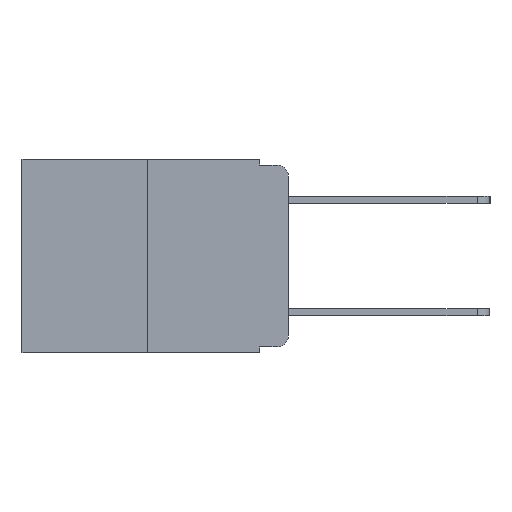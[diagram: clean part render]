
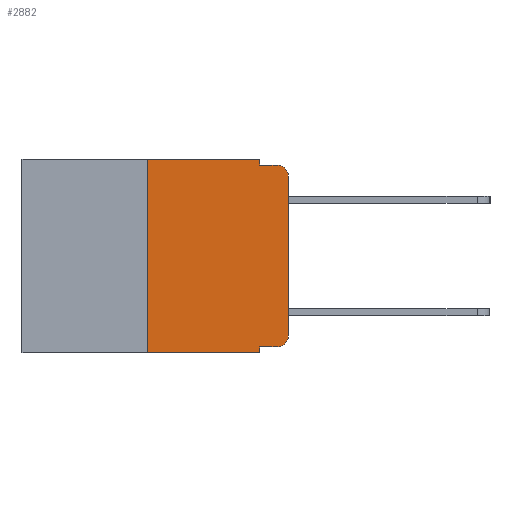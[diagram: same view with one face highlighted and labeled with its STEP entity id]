
A CAD part, left-side view. The second image highlights one B-rep face of the part: STEP entity #2882.
In plain terms, the highlighted planar face has unit normal (-1, 0, 0).
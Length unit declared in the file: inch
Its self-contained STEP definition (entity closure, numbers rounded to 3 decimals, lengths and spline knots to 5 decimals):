
#78 = FACE_OUTER_BOUND ( 'NONE', #7432, .T. ) ;
#578 = CARTESIAN_POINT ( 'NONE',  ( 0., 0.051, -0.343 ) ) ;
#594 = CARTESIAN_POINT ( 'NONE',  ( 0., 0.02, -0.01 ) ) ;
#706 = VECTOR ( 'NONE', #1500, 39.37008 ) ;
#825 = VERTEX_POINT ( 'NONE', #11015 ) ;
#967 = CARTESIAN_POINT ( 'NONE',  ( 0., 0.051, 0. ) ) ;
#990 = LINE ( 'NONE', #9850, #10139 ) ;
#1158 = VECTOR ( 'NONE', #1439, 39.37008 ) ;
#1318 = CARTESIAN_POINT ( 'NONE',  ( 0., 0.051, -0.333 ) ) ;
#1439 = DIRECTION ( 'NONE',  ( 0., -1., 0. ) ) ;
#1500 = DIRECTION ( 'NONE',  ( 0., -1., 0. ) ) ;
#1707 = VERTEX_POINT ( 'NONE', #967 ) ;
#2031 = EDGE_CURVE ( 'NONE', #7863, #6148, #9672, .T. ) ;
#2341 = PLANE ( 'NONE',  #5592 ) ;
#2882 = ADVANCED_FACE ( 'NONE', ( #78 ), #2341, .F. ) ;
#3167 = DIRECTION ( 'NONE',  ( -1., 0., 0. ) ) ;
#3210 = AXIS2_PLACEMENT_3D ( 'NONE', #8360, #3167, #9182 ) ;
#3216 = ORIENTED_EDGE ( 'NONE', *, *, #11448, .F. ) ;
#3262 = EDGE_CURVE ( 'NONE', #6536, #1707, #3329, .T. ) ;
#3329 = LINE ( 'NONE', #3497, #706 ) ;
#3354 = LINE ( 'NONE', #8130, #9667 ) ;
#3497 = CARTESIAN_POINT ( 'NONE',  ( 0., 0.473, 0. ) ) ;
#3505 = ORIENTED_EDGE ( 'NONE', *, *, #2031, .T. ) ;
#3533 = VECTOR ( 'NONE', #6987, 39.37008 ) ;
#3635 = VERTEX_POINT ( 'NONE', #5100 ) ;
#3747 = ORIENTED_EDGE ( 'NONE', *, *, #10014, .T. ) ;
#3861 = DIRECTION ( 'NONE',  ( 0., 0., -1. ) ) ;
#3976 = VECTOR ( 'NONE', #10927, 39.37008 ) ;
#4178 = LINE ( 'NONE', #5050, #8469 ) ;
#4180 = CARTESIAN_POINT ( 'NONE',  ( 0., 0.25, 0. ) ) ;
#4302 = ORIENTED_EDGE ( 'NONE', *, *, #10775, .F. ) ;
#4374 = DIRECTION ( 'NONE',  ( 1., 0., 0. ) ) ;
#4479 = DIRECTION ( 'NONE',  ( -1., 0., 0. ) ) ;
#4480 = CARTESIAN_POINT ( 'NONE',  ( 0., 0.02, -0.313 ) ) ;
#4847 = VERTEX_POINT ( 'NONE', #594 ) ;
#5050 = CARTESIAN_POINT ( 'NONE',  ( 0., 0.051, 0. ) ) ;
#5100 = CARTESIAN_POINT ( 'NONE',  ( 0., 0.051, -0.01 ) ) ;
#5101 = VERTEX_POINT ( 'NONE', #578 ) ;
#5106 = VECTOR ( 'NONE', #10142, 39.37008 ) ;
#5240 = DIRECTION ( 'NONE',  ( 0., 0., -1. ) ) ;
#5539 = ORIENTED_EDGE ( 'NONE', *, *, #8015, .T. ) ;
#5592 = AXIS2_PLACEMENT_3D ( 'NONE', #7612, #4374, #8631 ) ;
#5618 = EDGE_CURVE ( 'NONE', #8157, #6536, #9867, .T. ) ;
#6007 = CARTESIAN_POINT ( 'NONE',  ( 0., 0.473, -0.343 ) ) ;
#6047 = LINE ( 'NONE', #6007, #1158 ) ;
#6142 = CARTESIAN_POINT ( 'NONE',  ( 0., 0., 0. ) ) ;
#6148 = VERTEX_POINT ( 'NONE', #9809 ) ;
#6174 = EDGE_CURVE ( 'NONE', #825, #5101, #990, .T. ) ;
#6297 = LINE ( 'NONE', #1318, #3976 ) ;
#6396 = EDGE_CURVE ( 'NONE', #8157, #5101, #6047, .T. ) ;
#6413 = LINE ( 'NONE', #6142, #3533 ) ;
#6525 = ORIENTED_EDGE ( 'NONE', *, *, #6174, .F. ) ;
#6536 = VERTEX_POINT ( 'NONE', #11176 ) ;
#6728 = VERTEX_POINT ( 'NONE', #7178 ) ;
#6872 = ORIENTED_EDGE ( 'NONE', *, *, #5618, .F. ) ;
#6987 = DIRECTION ( 'NONE',  ( 0., 0., 1. ) ) ;
#7178 = CARTESIAN_POINT ( 'NONE',  ( 0., 0., -0.03 ) ) ;
#7296 = DIRECTION ( 'NONE',  ( 0., -1., 0. ) ) ;
#7432 = EDGE_LOOP ( 'NONE', ( #11473, #3747, #4302, #3216, #10449, #6872, #9623, #6525, #5539, #3505 ) ) ;
#7612 = CARTESIAN_POINT ( 'NONE',  ( 0., 0.473, 0. ) ) ;
#7863 = VERTEX_POINT ( 'NONE', #10009 ) ;
#8015 = EDGE_CURVE ( 'NONE', #825, #7863, #6297, .T. ) ;
#8130 = CARTESIAN_POINT ( 'NONE',  ( 0., 0.051, -0.01 ) ) ;
#8157 = VERTEX_POINT ( 'NONE', #8562 ) ;
#8360 = CARTESIAN_POINT ( 'NONE',  ( 0., 0.02, -0.03 ) ) ;
#8469 = VECTOR ( 'NONE', #9250, 39.37008 ) ;
#8562 = CARTESIAN_POINT ( 'NONE',  ( 0., 0.25, -0.343 ) ) ;
#8631 = DIRECTION ( 'NONE',  ( 0., 0., -1. ) ) ;
#9182 = DIRECTION ( 'NONE',  ( 0., 0., -1. ) ) ;
#9250 = DIRECTION ( 'NONE',  ( 0., 0., -1. ) ) ;
#9578 = EDGE_CURVE ( 'NONE', #6148, #6728, #6413, .T. ) ;
#9623 = ORIENTED_EDGE ( 'NONE', *, *, #6396, .T. ) ;
#9667 = VECTOR ( 'NONE', #7296, 39.37008 ) ;
#9672 = CIRCLE ( 'NONE', #10783, 0.02 ) ;
#9809 = CARTESIAN_POINT ( 'NONE',  ( 0., 0., -0.313 ) ) ;
#9850 = CARTESIAN_POINT ( 'NONE',  ( 0., 0.051, 0. ) ) ;
#9867 = LINE ( 'NONE', #4180, #5106 ) ;
#10009 = CARTESIAN_POINT ( 'NONE',  ( 0., 0.02, -0.333 ) ) ;
#10014 = EDGE_CURVE ( 'NONE', #6728, #4847, #11118, .T. ) ;
#10139 = VECTOR ( 'NONE', #3861, 39.37008 ) ;
#10142 = DIRECTION ( 'NONE',  ( 0., 0., 1. ) ) ;
#10449 = ORIENTED_EDGE ( 'NONE', *, *, #3262, .F. ) ;
#10775 = EDGE_CURVE ( 'NONE', #3635, #4847, #3354, .T. ) ;
#10783 = AXIS2_PLACEMENT_3D ( 'NONE', #4480, #4479, #5240 ) ;
#10927 = DIRECTION ( 'NONE',  ( 0., -1., 0. ) ) ;
#11015 = CARTESIAN_POINT ( 'NONE',  ( 0., 0.051, -0.333 ) ) ;
#11118 = CIRCLE ( 'NONE', #3210, 0.02 ) ;
#11176 = CARTESIAN_POINT ( 'NONE',  ( 0., 0.25, 0. ) ) ;
#11448 = EDGE_CURVE ( 'NONE', #1707, #3635, #4178, .T. ) ;
#11473 = ORIENTED_EDGE ( 'NONE', *, *, #9578, .T. ) ;
